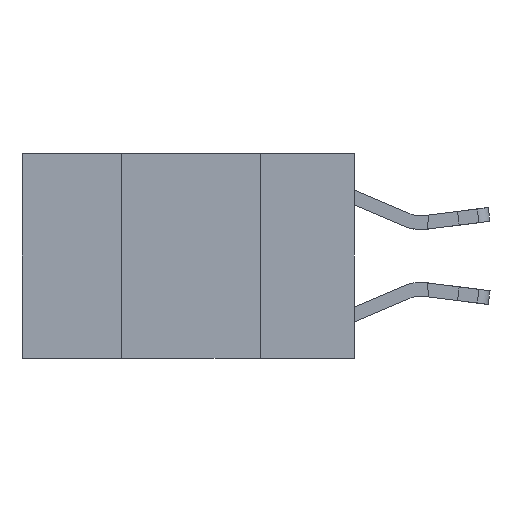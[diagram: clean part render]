
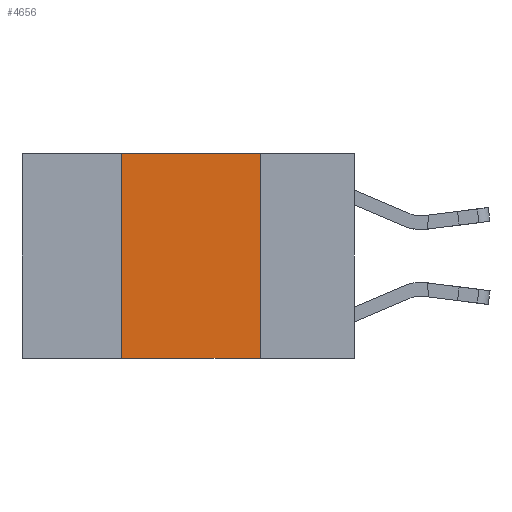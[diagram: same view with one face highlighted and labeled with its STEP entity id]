
A CAD part, left-side view. The second image highlights one B-rep face of the part: STEP entity #4656.
In plain terms, the highlighted planar face has unit normal (-1, 0, 0).
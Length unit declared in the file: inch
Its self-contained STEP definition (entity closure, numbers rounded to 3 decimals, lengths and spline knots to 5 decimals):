
#575 = EDGE_CURVE ( 'NONE', #1002, #10611, #4875, .T. ) ;
#801 = DIRECTION ( 'NONE',  ( 0., -1., 0. ) ) ;
#1002 = VERTEX_POINT ( 'NONE', #4716 ) ;
#1369 = PLANE ( 'NONE',  #14787 ) ;
#1912 = ORIENTED_EDGE ( 'NONE', *, *, #13998, .T. ) ;
#3056 = CARTESIAN_POINT ( 'NONE',  ( 0., 0.42, 0. ) ) ;
#4415 = DIRECTION ( 'NONE',  ( 1., 0., 0. ) ) ;
#4656 = ADVANCED_FACE ( 'NONE', ( #13851 ), #1369, .F. ) ;
#4716 = CARTESIAN_POINT ( 'NONE',  ( 0., 0.17, 0. ) ) ;
#4875 = LINE ( 'NONE', #18839, #16111 ) ;
#5445 = VECTOR ( 'NONE', #17287, 39.37008 ) ;
#5823 = CARTESIAN_POINT ( 'NONE',  ( 0., 0.6, 0. ) ) ;
#5972 = EDGE_CURVE ( 'NONE', #11197, #10469, #13567, .T. ) ;
#6318 = LINE ( 'NONE', #12599, #9765 ) ;
#6324 = ORIENTED_EDGE ( 'NONE', *, *, #5972, .F. ) ;
#7395 = DIRECTION ( 'NONE',  ( 0., 0., -1. ) ) ;
#7692 = CARTESIAN_POINT ( 'NONE',  ( 0., 0.42, 0. ) ) ;
#9265 = EDGE_LOOP ( 'NONE', ( #13244, #16654, #6324, #1912 ) ) ;
#9765 = VECTOR ( 'NONE', #801, 39.37008 ) ;
#10469 = VERTEX_POINT ( 'NONE', #3056 ) ;
#10611 = VERTEX_POINT ( 'NONE', #15127 ) ;
#11197 = VERTEX_POINT ( 'NONE', #15278 ) ;
#12599 = CARTESIAN_POINT ( 'NONE',  ( 0., 0.6, -0.37 ) ) ;
#13124 = VECTOR ( 'NONE', #14936, 39.37008 ) ;
#13244 = ORIENTED_EDGE ( 'NONE', *, *, #575, .F. ) ;
#13567 = LINE ( 'NONE', #7692, #13124 ) ;
#13851 = FACE_OUTER_BOUND ( 'NONE', #9265, .T. ) ;
#13998 = EDGE_CURVE ( 'NONE', #11197, #10611, #6318, .T. ) ;
#14412 = CARTESIAN_POINT ( 'NONE',  ( 0., 0.6, 0. ) ) ;
#14677 = DIRECTION ( 'NONE',  ( 0., 0., -1. ) ) ;
#14787 = AXIS2_PLACEMENT_3D ( 'NONE', #5823, #4415, #14677 ) ;
#14936 = DIRECTION ( 'NONE',  ( 0., 0., 1. ) ) ;
#15127 = CARTESIAN_POINT ( 'NONE',  ( 0., 0.17, -0.37 ) ) ;
#15278 = CARTESIAN_POINT ( 'NONE',  ( 0., 0.42, -0.37 ) ) ;
#16111 = VECTOR ( 'NONE', #7395, 39.37008 ) ;
#16654 = ORIENTED_EDGE ( 'NONE', *, *, #19060, .F. ) ;
#17128 = LINE ( 'NONE', #14412, #5445 ) ;
#17287 = DIRECTION ( 'NONE',  ( 0., -1., 0. ) ) ;
#18839 = CARTESIAN_POINT ( 'NONE',  ( 0., 0.17, 0. ) ) ;
#19060 = EDGE_CURVE ( 'NONE', #10469, #1002, #17128, .T. ) ;
